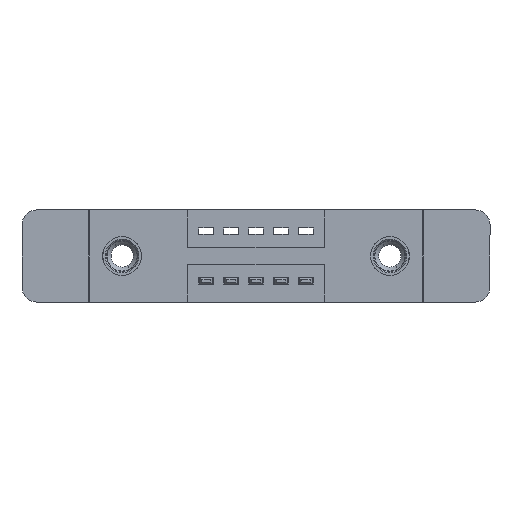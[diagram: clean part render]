
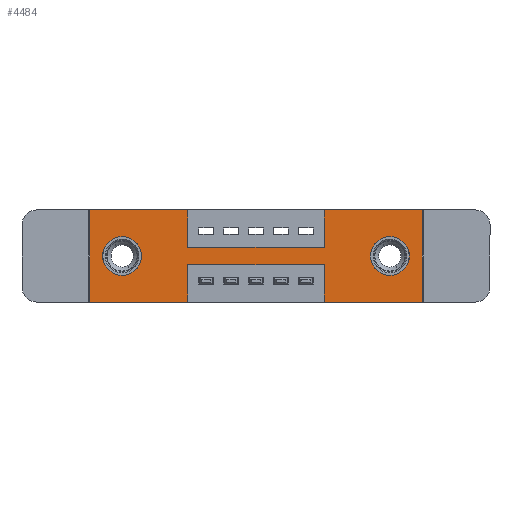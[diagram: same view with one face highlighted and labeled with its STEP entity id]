
A CAD part, front view. The second image highlights one B-rep face of the part: STEP entity #4484.
In plain terms, the highlighted planar face has unit normal (0, -1, 0).
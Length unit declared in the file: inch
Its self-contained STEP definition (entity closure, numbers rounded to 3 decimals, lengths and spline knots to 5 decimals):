
#91 = CARTESIAN_POINT ( 'NONE',  ( 0.13, 0., -0.185 ) ) ;
#106 = CARTESIAN_POINT ( 'NONE',  ( 0.13, 0., -0.185 ) ) ;
#112 = DIRECTION ( 'NONE',  ( 1., 0., 0. ) ) ;
#169 = ORIENTED_EDGE ( 'NONE', *, *, #6874, .T. ) ;
#452 = VERTEX_POINT ( 'NONE', #8351 ) ;
#498 = ORIENTED_EDGE ( 'NONE', *, *, #8444, .F. ) ;
#582 = DIRECTION ( 'NONE',  ( 1., 0., 0. ) ) ;
#710 = LINE ( 'NONE', #11149, #2670 ) ;
#839 = EDGE_CURVE ( 'NONE', #1956, #452, #8169, .T. ) ;
#869 = LINE ( 'NONE', #1344, #12311 ) ;
#909 = CIRCLE ( 'NONE', #9440, 0.078 ) ;
#1058 = VERTEX_POINT ( 'NONE', #11258 ) ;
#1109 = DIRECTION ( 'NONE',  ( 0., 0., 1. ) ) ;
#1289 = LINE ( 'NONE', #7395, #7534 ) ;
#1297 = DIRECTION ( 'NONE',  ( 0., 1., 0. ) ) ;
#1344 = CARTESIAN_POINT ( 'NONE',  ( 0.3925, 0., -0.37 ) ) ;
#1380 = ORIENTED_EDGE ( 'NONE', *, *, #12085, .F. ) ;
#1537 = DIRECTION ( 'NONE',  ( -1., 0., 0. ) ) ;
#1676 = CARTESIAN_POINT ( 'NONE',  ( 0.3925, 0., -0.22 ) ) ;
#1832 = CARTESIAN_POINT ( 'NONE',  ( 0.9425, 0., -0.37 ) ) ;
#1867 = EDGE_CURVE ( 'NONE', #7178, #9666, #909, .T. ) ;
#1956 = VERTEX_POINT ( 'NONE', #6406 ) ;
#1962 = VERTEX_POINT ( 'NONE', #2270 ) ;
#2089 = DIRECTION ( 'NONE',  ( 0., 1., 0. ) ) ;
#2185 = CARTESIAN_POINT ( 'NONE',  ( 0.3925, 0., -0.15 ) ) ;
#2254 = DIRECTION ( 'NONE',  ( 0., 0., 1. ) ) ;
#2270 = CARTESIAN_POINT ( 'NONE',  ( 0.3925, 0., 0. ) ) ;
#2373 = LINE ( 'NONE', #9660, #10491 ) ;
#2417 = EDGE_CURVE ( 'NONE', #13346, #7110, #6800, .T. ) ;
#2554 = EDGE_CURVE ( 'NONE', #452, #8556, #12826, .T. ) ;
#2670 = VECTOR ( 'NONE', #5873, 39.37008 ) ;
#3267 = ORIENTED_EDGE ( 'NONE', *, *, #6971, .F. ) ;
#3444 = EDGE_CURVE ( 'NONE', #1058, #1956, #869, .T. ) ;
#3467 = CARTESIAN_POINT ( 'NONE',  ( 0.9425, 0., -0.22 ) ) ;
#3783 = DIRECTION ( 'NONE',  ( -1., 0., 0. ) ) ;
#3855 = EDGE_CURVE ( 'NONE', #12635, #7830, #7941, .T. ) ;
#3902 = ORIENTED_EDGE ( 'NONE', *, *, #13458, .T. ) ;
#4207 = CARTESIAN_POINT ( 'NONE',  ( 0., 0., 0. ) ) ;
#4347 = DIRECTION ( 'NONE',  ( 0., 1., 0. ) ) ;
#4484 = ADVANCED_FACE ( 'NONE', ( #9779, #13625, #7928 ), #8180, .T. ) ;
#4494 = CARTESIAN_POINT ( 'NONE',  ( 0.13, 0., -0.107 ) ) ;
#4541 = CARTESIAN_POINT ( 'NONE',  ( 0., 0., -0.37 ) ) ;
#4867 = EDGE_LOOP ( 'NONE', ( #7120, #169 ) ) ;
#5164 = CARTESIAN_POINT ( 'NONE',  ( 1.205, 0., -0.263 ) ) ;
#5312 = LINE ( 'NONE', #2185, #11468 ) ;
#5705 = ORIENTED_EDGE ( 'NONE', *, *, #13716, .F. ) ;
#5739 = DIRECTION ( 'NONE',  ( 0., 0., 1. ) ) ;
#5740 = VECTOR ( 'NONE', #3783, 39.37008 ) ;
#5873 = DIRECTION ( 'NONE',  ( 0., 0., -1. ) ) ;
#5930 = EDGE_LOOP ( 'NONE', ( #3902, #7141 ) ) ;
#6231 = DIRECTION ( 'NONE',  ( 0., 0., 1. ) ) ;
#6406 = CARTESIAN_POINT ( 'NONE',  ( 0.3925, 0., -0.37 ) ) ;
#6780 = LINE ( 'NONE', #4207, #9300 ) ;
#6800 = CIRCLE ( 'NONE', #13211, 0.078 ) ;
#6874 = EDGE_CURVE ( 'NONE', #9666, #7178, #11511, .T. ) ;
#6948 = ORIENTED_EDGE ( 'NONE', *, *, #10652, .F. ) ;
#6960 = DIRECTION ( 'NONE',  ( 0., -1., 0. ) ) ;
#6971 = EDGE_CURVE ( 'NONE', #10256, #7541, #2373, .T. ) ;
#7110 = VERTEX_POINT ( 'NONE', #4494 ) ;
#7120 = ORIENTED_EDGE ( 'NONE', *, *, #1867, .T. ) ;
#7129 = VECTOR ( 'NONE', #5739, 39.37008 ) ;
#7141 = ORIENTED_EDGE ( 'NONE', *, *, #2417, .T. ) ;
#7178 = VERTEX_POINT ( 'NONE', #7702 ) ;
#7326 = VECTOR ( 'NONE', #1537, 39.37008 ) ;
#7369 = ORIENTED_EDGE ( 'NONE', *, *, #2554, .F. ) ;
#7395 = CARTESIAN_POINT ( 'NONE',  ( 1.335, 0., 0. ) ) ;
#7422 = DIRECTION ( 'NONE',  ( 0., 0., -1. ) ) ;
#7507 = ORIENTED_EDGE ( 'NONE', *, *, #3444, .F. ) ;
#7534 = VECTOR ( 'NONE', #9618, 39.37008 ) ;
#7541 = VERTEX_POINT ( 'NONE', #12659 ) ;
#7658 = CARTESIAN_POINT ( 'NONE',  ( 0.9425, 0., -0.37 ) ) ;
#7702 = CARTESIAN_POINT ( 'NONE',  ( 1.205, 0., -0.107 ) ) ;
#7741 = LINE ( 'NONE', #7658, #12262 ) ;
#7746 = VECTOR ( 'NONE', #582, 39.37008 ) ;
#7830 = VERTEX_POINT ( 'NONE', #1832 ) ;
#7845 = CARTESIAN_POINT ( 'NONE',  ( 0., 0., 0. ) ) ;
#7928 = FACE_OUTER_BOUND ( 'NONE', #12069, .T. ) ;
#7941 = LINE ( 'NONE', #12907, #10624 ) ;
#8129 = DIRECTION ( 'NONE',  ( 0., 0., -1. ) ) ;
#8169 = LINE ( 'NONE', #4541, #7326 ) ;
#8180 = PLANE ( 'NONE',  #13280 ) ;
#8203 = DIRECTION ( 'NONE',  ( 0., 0., -1. ) ) ;
#8331 = ORIENTED_EDGE ( 'NONE', *, *, #8578, .F. ) ;
#8351 = CARTESIAN_POINT ( 'NONE',  ( 0., 0., -0.37 ) ) ;
#8444 = EDGE_CURVE ( 'NONE', #12983, #10256, #5312, .T. ) ;
#8556 = VERTEX_POINT ( 'NONE', #11604 ) ;
#8578 = EDGE_CURVE ( 'NONE', #7541, #9413, #6780, .T. ) ;
#8652 = CARTESIAN_POINT ( 'NONE',  ( 1.205, 0., -0.185 ) ) ;
#8914 = CARTESIAN_POINT ( 'NONE',  ( 0., 0., 0. ) ) ;
#8915 = LINE ( 'NONE', #1676, #5740 ) ;
#8935 = DIRECTION ( 'NONE',  ( 0., 0., -1. ) ) ;
#8936 = LINE ( 'NONE', #7845, #7746 ) ;
#9300 = VECTOR ( 'NONE', #11651, 39.37008 ) ;
#9413 = VERTEX_POINT ( 'NONE', #11110 ) ;
#9440 = AXIS2_PLACEMENT_3D ( 'NONE', #8652, #4347, #7422 ) ;
#9618 = DIRECTION ( 'NONE',  ( 0., 0., -1. ) ) ;
#9660 = CARTESIAN_POINT ( 'NONE',  ( 0.9425, 0., 0. ) ) ;
#9666 = VERTEX_POINT ( 'NONE', #5164 ) ;
#9779 = FACE_BOUND ( 'NONE', #4867, .T. ) ;
#10153 = ORIENTED_EDGE ( 'NONE', *, *, #3855, .F. ) ;
#10190 = CARTESIAN_POINT ( 'NONE',  ( 0., 0., -0.37 ) ) ;
#10256 = VERTEX_POINT ( 'NONE', #12362 ) ;
#10444 = CARTESIAN_POINT ( 'NONE',  ( 1.205, 0., -0.185 ) ) ;
#10491 = VECTOR ( 'NONE', #1109, 39.37008 ) ;
#10624 = VECTOR ( 'NONE', #11935, 39.37008 ) ;
#10652 = EDGE_CURVE ( 'NONE', #7830, #12622, #7741, .T. ) ;
#10767 = CARTESIAN_POINT ( 'NONE',  ( 0.3925, 0., -0.15 ) ) ;
#11045 = EDGE_CURVE ( 'NONE', #12622, #1058, #8915, .T. ) ;
#11110 = CARTESIAN_POINT ( 'NONE',  ( 1.335, 0., 0. ) ) ;
#11149 = CARTESIAN_POINT ( 'NONE',  ( 0.3925, 0., 0. ) ) ;
#11258 = CARTESIAN_POINT ( 'NONE',  ( 0.3925, 0., -0.22 ) ) ;
#11341 = ORIENTED_EDGE ( 'NONE', *, *, #11845, .F. ) ;
#11468 = VECTOR ( 'NONE', #112, 39.37008 ) ;
#11511 = CIRCLE ( 'NONE', #12507, 0.078 ) ;
#11604 = CARTESIAN_POINT ( 'NONE',  ( 0., 0., 0. ) ) ;
#11651 = DIRECTION ( 'NONE',  ( 1., 0., 0. ) ) ;
#11842 = DIRECTION ( 'NONE',  ( 0., 0., 1. ) ) ;
#11845 = EDGE_CURVE ( 'NONE', #9413, #12635, #1289, .T. ) ;
#11930 = AXIS2_PLACEMENT_3D ( 'NONE', #106, #2089, #6231 ) ;
#11935 = DIRECTION ( 'NONE',  ( -1., 0., 0. ) ) ;
#11978 = CARTESIAN_POINT ( 'NONE',  ( 1.335, 0., -0.37 ) ) ;
#12069 = EDGE_LOOP ( 'NONE', ( #7507, #12829, #6948, #10153, #11341, #8331, #3267, #498, #1380, #5705, #7369, #12587 ) ) ;
#12085 = EDGE_CURVE ( 'NONE', #1962, #12983, #710, .T. ) ;
#12262 = VECTOR ( 'NONE', #11842, 39.37008 ) ;
#12311 = VECTOR ( 'NONE', #8935, 39.37008 ) ;
#12362 = CARTESIAN_POINT ( 'NONE',  ( 0.9425, 0., -0.15 ) ) ;
#12507 = AXIS2_PLACEMENT_3D ( 'NONE', #10444, #12646, #8203 ) ;
#12540 = CARTESIAN_POINT ( 'NONE',  ( 0.13, 0., -0.263 ) ) ;
#12587 = ORIENTED_EDGE ( 'NONE', *, *, #839, .F. ) ;
#12622 = VERTEX_POINT ( 'NONE', #3467 ) ;
#12635 = VERTEX_POINT ( 'NONE', #11978 ) ;
#12646 = DIRECTION ( 'NONE',  ( 0., 1., 0. ) ) ;
#12659 = CARTESIAN_POINT ( 'NONE',  ( 0.9425, 0., 0. ) ) ;
#12826 = LINE ( 'NONE', #8914, #7129 ) ;
#12829 = ORIENTED_EDGE ( 'NONE', *, *, #11045, .F. ) ;
#12907 = CARTESIAN_POINT ( 'NONE',  ( 0., 0., -0.37 ) ) ;
#12983 = VERTEX_POINT ( 'NONE', #10767 ) ;
#13211 = AXIS2_PLACEMENT_3D ( 'NONE', #91, #1297, #2254 ) ;
#13280 = AXIS2_PLACEMENT_3D ( 'NONE', #10190, #6960, #8129 ) ;
#13288 = CIRCLE ( 'NONE', #11930, 0.078 ) ;
#13346 = VERTEX_POINT ( 'NONE', #12540 ) ;
#13458 = EDGE_CURVE ( 'NONE', #7110, #13346, #13288, .T. ) ;
#13625 = FACE_BOUND ( 'NONE', #5930, .T. ) ;
#13716 = EDGE_CURVE ( 'NONE', #8556, #1962, #8936, .T. ) ;
